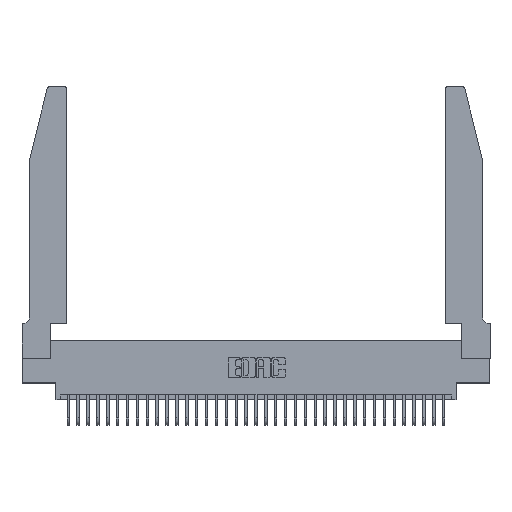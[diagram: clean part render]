
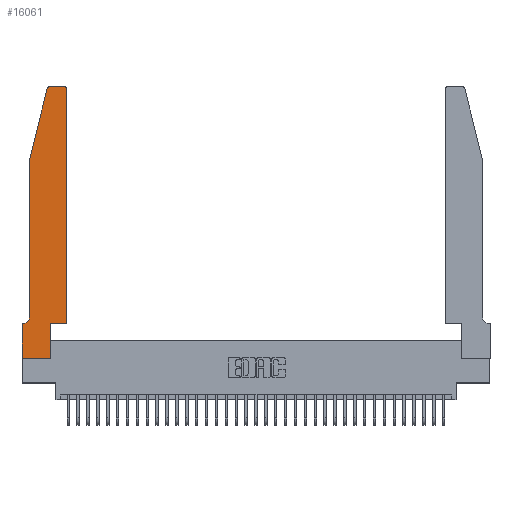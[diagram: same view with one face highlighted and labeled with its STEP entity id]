
A CAD part, top view. The second image highlights one B-rep face of the part: STEP entity #16061.
In plain terms, the highlighted planar face has unit normal (0, 0, 1).
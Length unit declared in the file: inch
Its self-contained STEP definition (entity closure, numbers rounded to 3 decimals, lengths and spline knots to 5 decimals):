
#97 = DIRECTION ( 'NONE',  ( -1., 0., 0. ) ) ;
#140 = CIRCLE ( 'NONE', #15722, 0.03 ) ;
#448 = VERTEX_POINT ( 'NONE', #15164 ) ;
#725 = ORIENTED_EDGE ( 'NONE', *, *, #30402, .T. ) ;
#1105 = VECTOR ( 'NONE', #27365, 39.37008 ) ;
#1142 = CARTESIAN_POINT ( 'NONE',  ( 0.284, 2.75, 0.37 ) ) ;
#1152 = CARTESIAN_POINT ( 'NONE',  ( 0., 0., 0.37 ) ) ;
#2456 = CARTESIAN_POINT ( 'NONE',  ( 0., 0.35, 0.37 ) ) ;
#2708 = CARTESIAN_POINT ( 'NONE',  ( 0.2865, 0.35, 0.37 ) ) ;
#3045 = LINE ( 'NONE', #1152, #11148 ) ;
#3182 = ORIENTED_EDGE ( 'NONE', *, *, #7098, .T. ) ;
#3509 = CARTESIAN_POINT ( 'NONE',  ( 0.4505, 2.72, 0.37 ) ) ;
#3860 = VERTEX_POINT ( 'NONE', #29181 ) ;
#4698 = EDGE_LOOP ( 'NONE', ( #17389, #13497, #22057, #725, #31990, #6821, #14575, #13862, #31325, #3182, #26108, #23993 ) ) ;
#4909 = DIRECTION ( 'NONE',  ( 0., 0., 1. ) ) ;
#4998 = CARTESIAN_POINT ( 'NONE',  ( 0.2605, 2.75, 0.37 ) ) ;
#5452 = DIRECTION ( 'NONE',  ( 0., 1., 0. ) ) ;
#5715 = DIRECTION ( 'NONE',  ( 0., 0., 1. ) ) ;
#5756 = CARTESIAN_POINT ( 'NONE',  ( 0.4505, 0.35, 0.37 ) ) ;
#6310 = VERTEX_POINT ( 'NONE', #32737 ) ;
#6606 = LINE ( 'NONE', #19876, #20019 ) ;
#6693 = DIRECTION ( 'NONE',  ( 1., 0., 0. ) ) ;
#6821 = ORIENTED_EDGE ( 'NONE', *, *, #32344, .T. ) ;
#7098 = EDGE_CURVE ( 'NONE', #448, #6310, #34476, .T. ) ;
#7220 = EDGE_CURVE ( 'NONE', #34662, #15481, #31148, .T. ) ;
#7770 = DIRECTION ( 'NONE',  ( -1., 0., 0. ) ) ;
#7823 = VECTOR ( 'NONE', #8950, 39.37008 ) ;
#8822 = CARTESIAN_POINT ( 'NONE',  ( 0.2865, 0., 0.37 ) ) ;
#8950 = DIRECTION ( 'NONE',  ( 1., 0., 0. ) ) ;
#9457 = EDGE_CURVE ( 'NONE', #15481, #11288, #3045, .T. ) ;
#9645 = CARTESIAN_POINT ( 'NONE',  ( 0., 0., 0.37 ) ) ;
#9867 = EDGE_CURVE ( 'NONE', #11288, #448, #26056, .T. ) ;
#10686 = DIRECTION ( 'NONE',  ( 0., 0., 1. ) ) ;
#10864 = CARTESIAN_POINT ( 'NONE',  ( 0.0055, 0.42, 0.37 ) ) ;
#11119 = VECTOR ( 'NONE', #5452, 39.37008 ) ;
#11148 = VECTOR ( 'NONE', #6693, 39.37008 ) ;
#11207 = FACE_OUTER_BOUND ( 'NONE', #4698, .T. ) ;
#11288 = VERTEX_POINT ( 'NONE', #8822 ) ;
#11409 = LINE ( 'NONE', #4998, #24681 ) ;
#11439 = VERTEX_POINT ( 'NONE', #1142 ) ;
#11470 = EDGE_CURVE ( 'NONE', #30204, #3860, #31791, .T. ) ;
#11511 = AXIS2_PLACEMENT_3D ( 'NONE', #10864, #29457, #13566 ) ;
#12122 = VERTEX_POINT ( 'NONE', #22243 ) ;
#13497 = ORIENTED_EDGE ( 'NONE', *, *, #17241, .T. ) ;
#13566 = DIRECTION ( 'NONE',  ( -1., 0., 0. ) ) ;
#13731 = EDGE_CURVE ( 'NONE', #12122, #32059, #23322, .T. ) ;
#13862 = ORIENTED_EDGE ( 'NONE', *, *, #9457, .T. ) ;
#14470 = CIRCLE ( 'NONE', #30199, 0.03 ) ;
#14575 = ORIENTED_EDGE ( 'NONE', *, *, #7220, .T. ) ;
#15164 = CARTESIAN_POINT ( 'NONE',  ( 0.2865, 0.35, 0.37 ) ) ;
#15372 = VECTOR ( 'NONE', #97, 39.37008 ) ;
#15481 = VERTEX_POINT ( 'NONE', #18785 ) ;
#15569 = EDGE_CURVE ( 'NONE', #23309, #28608, #140, .T. ) ;
#15722 = AXIS2_PLACEMENT_3D ( 'NONE', #21750, #5715, #24403 ) ;
#16061 = ADVANCED_FACE ( 'NONE', ( #11207 ), #26597, .T. ) ;
#16343 = CARTESIAN_POINT ( 'NONE',  ( 0.0755, 0.35, 0.37 ) ) ;
#17040 = VECTOR ( 'NONE', #33599, 39.37008 ) ;
#17241 = EDGE_CURVE ( 'NONE', #11439, #30204, #14470, .T. ) ;
#17389 = ORIENTED_EDGE ( 'NONE', *, *, #19542, .T. ) ;
#18785 = CARTESIAN_POINT ( 'NONE',  ( 0., 0., 0.37 ) ) ;
#19542 = EDGE_CURVE ( 'NONE', #28608, #11439, #11409, .T. ) ;
#19876 = CARTESIAN_POINT ( 'NONE',  ( 0.0755, 2., 0.37 ) ) ;
#20019 = VECTOR ( 'NONE', #22492, 39.37008 ) ;
#20990 = CARTESIAN_POINT ( 'NONE',  ( 0.284, 2.72, 0.37 ) ) ;
#21750 = CARTESIAN_POINT ( 'NONE',  ( 0.4205, 2.72, 0.37 ) ) ;
#22057 = ORIENTED_EDGE ( 'NONE', *, *, #11470, .T. ) ;
#22243 = CARTESIAN_POINT ( 'NONE',  ( 0.0755, 0.42, 0.37 ) ) ;
#22492 = DIRECTION ( 'NONE',  ( 0., -1., 0. ) ) ;
#23207 = LINE ( 'NONE', #16343, #15372 ) ;
#23309 = VERTEX_POINT ( 'NONE', #3509 ) ;
#23322 = CIRCLE ( 'NONE', #11511, 0.07 ) ;
#23626 = DIRECTION ( 'NONE',  ( 1., 0., 0. ) ) ;
#23854 = VECTOR ( 'NONE', #30706, 39.37008 ) ;
#23993 = ORIENTED_EDGE ( 'NONE', *, *, #15569, .T. ) ;
#24241 = CARTESIAN_POINT ( 'NONE',  ( 0.25487, 2.72718, 0.37 ) ) ;
#24403 = DIRECTION ( 'NONE',  ( 1., 0., 0. ) ) ;
#24681 = VECTOR ( 'NONE', #7770, 39.37008 ) ;
#26056 = LINE ( 'NONE', #2708, #11119 ) ;
#26108 = ORIENTED_EDGE ( 'NONE', *, *, #29068, .T. ) ;
#26597 = PLANE ( 'NONE',  #32848 ) ;
#27365 = DIRECTION ( 'NONE',  ( 0., 1., 0. ) ) ;
#27563 = CARTESIAN_POINT ( 'NONE',  ( 0.4505, 0.35, 0.37 ) ) ;
#27758 = CARTESIAN_POINT ( 'NONE',  ( 0.4205, 2.75, 0.37 ) ) ;
#28234 = CARTESIAN_POINT ( 'NONE',  ( 0., 0.35, 0.37 ) ) ;
#28608 = VERTEX_POINT ( 'NONE', #27758 ) ;
#29068 = EDGE_CURVE ( 'NONE', #6310, #23309, #34208, .T. ) ;
#29181 = CARTESIAN_POINT ( 'NONE',  ( 0.0755, 2., 0.37 ) ) ;
#29273 = DIRECTION ( 'NONE',  ( 1., 0., 0. ) ) ;
#29457 = DIRECTION ( 'NONE',  ( 0., 0., -1. ) ) ;
#30199 = AXIS2_PLACEMENT_3D ( 'NONE', #20990, #4909, #23626 ) ;
#30204 = VERTEX_POINT ( 'NONE', #24241 ) ;
#30402 = EDGE_CURVE ( 'NONE', #3860, #12122, #6606, .T. ) ;
#30706 = DIRECTION ( 'NONE',  ( -0.239, -0.971, 0. ) ) ;
#31148 = LINE ( 'NONE', #9645, #17040 ) ;
#31325 = ORIENTED_EDGE ( 'NONE', *, *, #9867, .T. ) ;
#31791 = LINE ( 'NONE', #33369, #23854 ) ;
#31990 = ORIENTED_EDGE ( 'NONE', *, *, #13731, .T. ) ;
#32059 = VERTEX_POINT ( 'NONE', #33634 ) ;
#32344 = EDGE_CURVE ( 'NONE', #32059, #34662, #23207, .T. ) ;
#32737 = CARTESIAN_POINT ( 'NONE',  ( 0.4505, 0.35, 0.37 ) ) ;
#32848 = AXIS2_PLACEMENT_3D ( 'NONE', #2456, #10686, #29273 ) ;
#33369 = CARTESIAN_POINT ( 'NONE',  ( 0.0755, 2., 0.37 ) ) ;
#33599 = DIRECTION ( 'NONE',  ( 0., -1., 0. ) ) ;
#33634 = CARTESIAN_POINT ( 'NONE',  ( 0.0055, 0.35, 0.37 ) ) ;
#34208 = LINE ( 'NONE', #5756, #1105 ) ;
#34476 = LINE ( 'NONE', #27563, #7823 ) ;
#34662 = VERTEX_POINT ( 'NONE', #28234 ) ;
